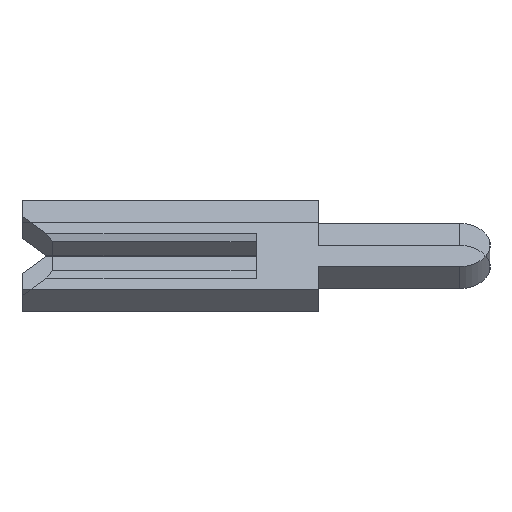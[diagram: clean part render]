
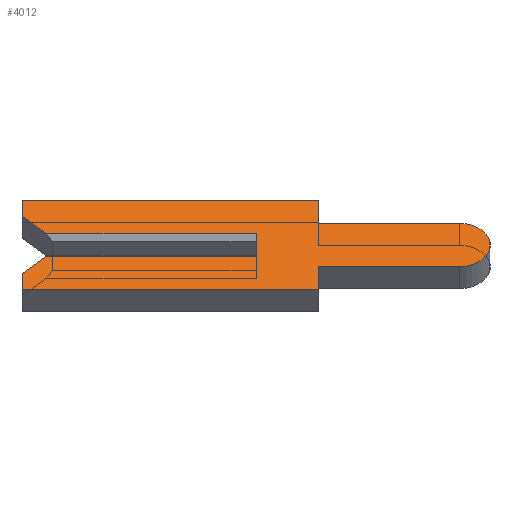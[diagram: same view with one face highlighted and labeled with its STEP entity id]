
A CAD part, left-side view. The second image highlights one B-rep face of the part: STEP entity #4012.
In plain terms, the highlighted face is planar.
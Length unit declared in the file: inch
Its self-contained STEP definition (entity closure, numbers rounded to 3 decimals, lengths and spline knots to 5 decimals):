
#32 = LINE ( 'NONE', #1828, #580 ) ;
#86 = CARTESIAN_POINT ( 'NONE',  ( -0.01, 0.15, -0.026 ) ) ;
#135 = CARTESIAN_POINT ( 'NONE',  ( -0.01, -0.04, 0.04 ) ) ;
#145 = VERTEX_POINT ( 'NONE', #2702 ) ;
#219 = ORIENTED_EDGE ( 'NONE', *, *, #1422, .F. ) ;
#279 = CARTESIAN_POINT ( 'NONE',  ( -0.01, 0.1305, -0.0065 ) ) ;
#305 = CARTESIAN_POINT ( 'NONE',  ( -0.01, -0.1305, -0.01 ) ) ;
#323 = EDGE_LOOP ( 'NONE', ( #2811, #3768, #3116, #4112, #3387, #3086, #2749, #1062, #562, #2797, #219, #1064, #3881, #1205 ) ) ;
#350 = DIRECTION ( 'NONE',  ( 0., -1., 0. ) ) ;
#400 = CARTESIAN_POINT ( 'NONE',  ( -0.01, 0.15, -0.026 ) ) ;
#464 = LINE ( 'NONE', #3031, #567 ) ;
#491 = DIRECTION ( 'NONE',  ( 0., 0., -1. ) ) ;
#562 = ORIENTED_EDGE ( 'NONE', *, *, #3407, .F. ) ;
#563 = LINE ( 'NONE', #1022, #1831 ) ;
#567 = VECTOR ( 'NONE', #3713, 39.37008 ) ;
#580 = VECTOR ( 'NONE', #4203, 39.37008 ) ;
#623 = AXIS2_PLACEMENT_3D ( 'NONE', #2623, #3376, #1956 ) ;
#651 = EDGE_CURVE ( 'NONE', #3246, #1059, #1347, .T. ) ;
#753 = CARTESIAN_POINT ( 'NONE',  ( -0.01, 0.15, 0.026 ) ) ;
#774 = LINE ( 'NONE', #2083, #2455 ) ;
#776 = CARTESIAN_POINT ( 'NONE',  ( -0.01, -0.04, -0.0195 ) ) ;
#784 = VERTEX_POINT ( 'NONE', #3453 ) ;
#817 = EDGE_CURVE ( 'NONE', #1264, #2627, #3830, .T. ) ;
#913 = CARTESIAN_POINT ( 'NONE',  ( -0.01, -0.04, 0.04 ) ) ;
#967 = DIRECTION ( 'NONE',  ( 0., 1., 0. ) ) ;
#1022 = CARTESIAN_POINT ( 'NONE',  ( -0.01, 0.15, 0.01 ) ) ;
#1034 = CIRCLE ( 'NONE', #623, 0.0195 ) ;
#1059 = VERTEX_POINT ( 'NONE', #400 ) ;
#1062 = ORIENTED_EDGE ( 'NONE', *, *, #3864, .F. ) ;
#1064 = ORIENTED_EDGE ( 'NONE', *, *, #4023, .F. ) ;
#1094 = VERTEX_POINT ( 'NONE', #776 ) ;
#1098 = VECTOR ( 'NONE', #491, 39.37008 ) ;
#1205 = ORIENTED_EDGE ( 'NONE', *, *, #1535, .F. ) ;
#1264 = VERTEX_POINT ( 'NONE', #3799 ) ;
#1310 = VERTEX_POINT ( 'NONE', #4126 ) ;
#1314 = VECTOR ( 'NONE', #1423, 39.37008 ) ;
#1318 = CARTESIAN_POINT ( 'NONE',  ( -0.01, -0.1305, 0. ) ) ;
#1347 = LINE ( 'NONE', #86, #3307 ) ;
#1422 = EDGE_CURVE ( 'NONE', #3926, #3302, #1912, .T. ) ;
#1423 = DIRECTION ( 'NONE',  ( 0., 0., 1. ) ) ;
#1453 = EDGE_CURVE ( 'NONE', #145, #784, #3786, .T. ) ;
#1473 = LINE ( 'NONE', #1659, #3956 ) ;
#1484 = CARTESIAN_POINT ( 'NONE',  ( -0.01, -0.04, -0.04 ) ) ;
#1517 = CARTESIAN_POINT ( 'NONE',  ( -0.01, 0.1305, 0.0065 ) ) ;
#1535 = EDGE_CURVE ( 'NONE', #3778, #1264, #4014, .T. ) ;
#1581 = VECTOR ( 'NONE', #3336, 39.37008 ) ;
#1592 = CARTESIAN_POINT ( 'NONE',  ( -0.01, -0.04, 0.0195 ) ) ;
#1659 = CARTESIAN_POINT ( 'NONE',  ( -0.01, -0.04, -0.0195 ) ) ;
#1674 = EDGE_CURVE ( 'NONE', #1841, #3246, #32, .T. ) ;
#1681 = CARTESIAN_POINT ( 'NONE',  ( -0.01, 0.134, 0.01 ) ) ;
#1757 = DIRECTION ( 'NONE',  ( 0., 0., 1. ) ) ;
#1803 = VERTEX_POINT ( 'NONE', #2885 ) ;
#1828 = CARTESIAN_POINT ( 'NONE',  ( -0.01, 0.15, -0.04 ) ) ;
#1831 = VECTOR ( 'NONE', #350, 39.37008 ) ;
#1841 = VERTEX_POINT ( 'NONE', #1484 ) ;
#1912 = LINE ( 'NONE', #135, #1098 ) ;
#1956 = DIRECTION ( 'NONE',  ( 0., 0., -1. ) ) ;
#2071 = VERTEX_POINT ( 'NONE', #4215 ) ;
#2083 = CARTESIAN_POINT ( 'NONE',  ( -0.01, -0.04, -0.04 ) ) ;
#2167 = DIRECTION ( 'NONE',  ( 0., 0.707, 0.707 ) ) ;
#2186 = CARTESIAN_POINT ( 'NONE',  ( -0.01, 0., 0.0065 ) ) ;
#2209 = VECTOR ( 'NONE', #2167, 39.37008 ) ;
#2310 = DIRECTION ( 'NONE',  ( 0., -1., 0. ) ) ;
#2355 = LINE ( 'NONE', #305, #3645 ) ;
#2455 = VECTOR ( 'NONE', #4009, 39.37008 ) ;
#2547 = CARTESIAN_POINT ( 'NONE',  ( -0.01, 0.15, 0.04 ) ) ;
#2623 = CARTESIAN_POINT ( 'NONE',  ( -0.01, -0.1305, 0. ) ) ;
#2627 = VERTEX_POINT ( 'NONE', #2547 ) ;
#2702 = CARTESIAN_POINT ( 'NONE',  ( -0.01, 0., -0.01 ) ) ;
#2749 = ORIENTED_EDGE ( 'NONE', *, *, #3549, .F. ) ;
#2786 = FACE_OUTER_BOUND ( 'NONE', #323, .T. ) ;
#2797 = ORIENTED_EDGE ( 'NONE', *, *, #2926, .F. ) ;
#2811 = ORIENTED_EDGE ( 'NONE', *, *, #4250, .T. ) ;
#2834 = DIRECTION ( 'NONE',  ( 0., 0., 1. ) ) ;
#2875 = VECTOR ( 'NONE', #2834, 39.37008 ) ;
#2885 = CARTESIAN_POINT ( 'NONE',  ( -0.01, 0.134, -0.01 ) ) ;
#2926 = EDGE_CURVE ( 'NONE', #3302, #2071, #3856, .T. ) ;
#2932 = DIRECTION ( 'NONE',  ( 0., -1., 0. ) ) ;
#3031 = CARTESIAN_POINT ( 'NONE',  ( -0.01, 0.15, 0.04 ) ) ;
#3086 = ORIENTED_EDGE ( 'NONE', *, *, #1674, .F. ) ;
#3116 = ORIENTED_EDGE ( 'NONE', *, *, #3718, .F. ) ;
#3117 = LINE ( 'NONE', #279, #1581 ) ;
#3246 = VERTEX_POINT ( 'NONE', #3599 ) ;
#3302 = VERTEX_POINT ( 'NONE', #3586 ) ;
#3307 = VECTOR ( 'NONE', #1757, 39.37008 ) ;
#3336 = DIRECTION ( 'NONE',  ( 0., -0.707, 0.707 ) ) ;
#3350 = PLANE ( 'NONE',  #4055 ) ;
#3376 = DIRECTION ( 'NONE',  ( 1., 0., 0. ) ) ;
#3387 = ORIENTED_EDGE ( 'NONE', *, *, #651, .F. ) ;
#3407 = EDGE_CURVE ( 'NONE', #2071, #1310, #1034, .T. ) ;
#3453 = CARTESIAN_POINT ( 'NONE',  ( -0.01, 0., 0.01 ) ) ;
#3549 = EDGE_CURVE ( 'NONE', #1094, #1841, #774, .T. ) ;
#3586 = CARTESIAN_POINT ( 'NONE',  ( -0.01, -0.04, 0.0195 ) ) ;
#3599 = CARTESIAN_POINT ( 'NONE',  ( -0.01, 0.15, -0.04 ) ) ;
#3645 = VECTOR ( 'NONE', #2310, 39.37008 ) ;
#3701 = DIRECTION ( 'NONE',  ( 0., 0., -1. ) ) ;
#3713 = DIRECTION ( 'NONE',  ( 0., -1., 0. ) ) ;
#3718 = EDGE_CURVE ( 'NONE', #1803, #145, #2355, .T. ) ;
#3768 = ORIENTED_EDGE ( 'NONE', *, *, #1453, .F. ) ;
#3778 = VERTEX_POINT ( 'NONE', #1681 ) ;
#3786 = LINE ( 'NONE', #2186, #2875 ) ;
#3799 = CARTESIAN_POINT ( 'NONE',  ( -0.01, 0.15, 0.026 ) ) ;
#3830 = LINE ( 'NONE', #753, #1314 ) ;
#3856 = LINE ( 'NONE', #1592, #3860 ) ;
#3860 = VECTOR ( 'NONE', #2932, 39.37008 ) ;
#3864 = EDGE_CURVE ( 'NONE', #1310, #1094, #1473, .T. ) ;
#3881 = ORIENTED_EDGE ( 'NONE', *, *, #817, .F. ) ;
#3926 = VERTEX_POINT ( 'NONE', #913 ) ;
#3956 = VECTOR ( 'NONE', #967, 39.37008 ) ;
#4009 = DIRECTION ( 'NONE',  ( 0., 0., -1. ) ) ;
#4012 = ADVANCED_FACE ( 'NONE', ( #2786 ), #3350, .F. ) ;
#4014 = LINE ( 'NONE', #1517, #2209 ) ;
#4019 = DIRECTION ( 'NONE',  ( 1., 0., 0. ) ) ;
#4023 = EDGE_CURVE ( 'NONE', #2627, #3926, #464, .T. ) ;
#4055 = AXIS2_PLACEMENT_3D ( 'NONE', #1318, #4019, #3701 ) ;
#4109 = EDGE_CURVE ( 'NONE', #1059, #1803, #3117, .T. ) ;
#4112 = ORIENTED_EDGE ( 'NONE', *, *, #4109, .F. ) ;
#4126 = CARTESIAN_POINT ( 'NONE',  ( -0.01, -0.1305, -0.0195 ) ) ;
#4203 = DIRECTION ( 'NONE',  ( 0., 1., 0. ) ) ;
#4215 = CARTESIAN_POINT ( 'NONE',  ( -0.01, -0.1305, 0.0195 ) ) ;
#4250 = EDGE_CURVE ( 'NONE', #3778, #784, #563, .T. ) ;
